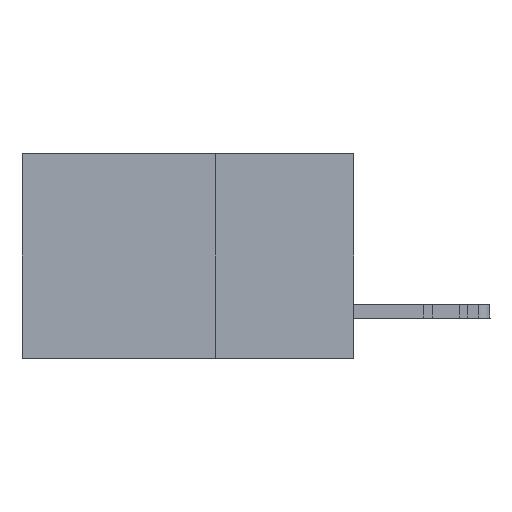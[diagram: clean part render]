
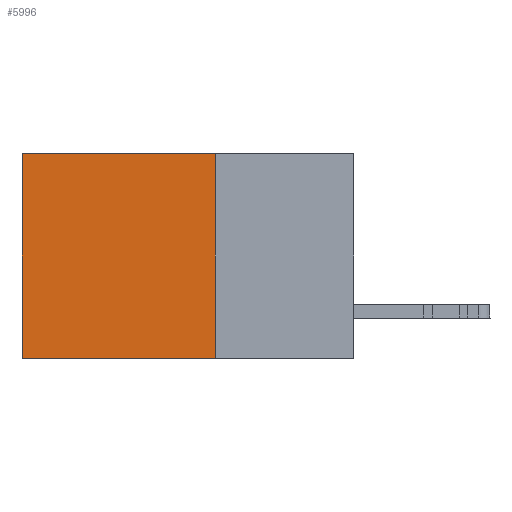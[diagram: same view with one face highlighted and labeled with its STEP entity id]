
A CAD part, left-side view. The second image highlights one B-rep face of the part: STEP entity #5996.
In plain terms, the highlighted planar face has unit normal (-1, 0, 0).
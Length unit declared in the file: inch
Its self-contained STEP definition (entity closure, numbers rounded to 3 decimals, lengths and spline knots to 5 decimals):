
#2182 = CARTESIAN_POINT ( 'NONE',  ( 0.2875, 0.25, -0.37 ) ) ;
#2769 = ORIENTED_EDGE ( 'NONE', *, *, #18118, .T. ) ;
#3696 = DIRECTION ( 'NONE',  ( 0., 0., -1. ) ) ;
#4790 = CARTESIAN_POINT ( 'NONE',  ( 0.2875, 0.25, 0. ) ) ;
#5996 = ADVANCED_FACE ( 'NONE', ( #18856 ), #25806, .F. ) ;
#6722 = CARTESIAN_POINT ( 'NONE',  ( 0.2875, 0.25, -0.37 ) ) ;
#7724 = DIRECTION ( 'NONE',  ( 0., 0., -1. ) ) ;
#10434 = CARTESIAN_POINT ( 'NONE',  ( 0.2875, 0.6, 0. ) ) ;
#10966 = VERTEX_POINT ( 'NONE', #10434 ) ;
#14449 = DIRECTION ( 'NONE',  ( 1., 0., 0. ) ) ;
#16374 = ORIENTED_EDGE ( 'NONE', *, *, #29642, .F. ) ;
#16858 = LINE ( 'NONE', #6722, #21499 ) ;
#17360 = ORIENTED_EDGE ( 'NONE', *, *, #20491, .F. ) ;
#18118 = EDGE_CURVE ( 'NONE', #10966, #45954, #29703, .T. ) ;
#18443 = CARTESIAN_POINT ( 'NONE',  ( 0.2875, 0.25, 0. ) ) ;
#18856 = FACE_OUTER_BOUND ( 'NONE', #36095, .T. ) ;
#20147 = CARTESIAN_POINT ( 'NONE',  ( 0.2875, 0.6, 0. ) ) ;
#20491 = EDGE_CURVE ( 'NONE', #46075, #43685, #34114, .T. ) ;
#21499 = VECTOR ( 'NONE', #36011, 39.37008 ) ;
#23917 = VECTOR ( 'NONE', #38473, 39.37008 ) ;
#24671 = CARTESIAN_POINT ( 'NONE',  ( 0.2875, 0.25, 0. ) ) ;
#25806 = PLANE ( 'NONE',  #40801 ) ;
#27270 = CARTESIAN_POINT ( 'NONE',  ( 0.2875, 0.6, -0.37 ) ) ;
#29283 = EDGE_CURVE ( 'NONE', #46075, #10966, #33214, .T. ) ;
#29642 = EDGE_CURVE ( 'NONE', #43685, #45954, #16858, .T. ) ;
#29703 = LINE ( 'NONE', #20147, #41432 ) ;
#31388 = DIRECTION ( 'NONE',  ( 0., 0., -1. ) ) ;
#33030 = ORIENTED_EDGE ( 'NONE', *, *, #29283, .T. ) ;
#33214 = LINE ( 'NONE', #4790, #23917 ) ;
#34114 = LINE ( 'NONE', #18443, #38155 ) ;
#36011 = DIRECTION ( 'NONE',  ( 0., 1., 0. ) ) ;
#36095 = EDGE_LOOP ( 'NONE', ( #2769, #16374, #17360, #33030 ) ) ;
#38155 = VECTOR ( 'NONE', #7724, 39.37008 ) ;
#38473 = DIRECTION ( 'NONE',  ( 0., 1., 0. ) ) ;
#40801 = AXIS2_PLACEMENT_3D ( 'NONE', #44550, #14449, #3696 ) ;
#41432 = VECTOR ( 'NONE', #31388, 39.37008 ) ;
#43685 = VERTEX_POINT ( 'NONE', #2182 ) ;
#44550 = CARTESIAN_POINT ( 'NONE',  ( 0.2875, 0.25, 0. ) ) ;
#45954 = VERTEX_POINT ( 'NONE', #27270 ) ;
#46075 = VERTEX_POINT ( 'NONE', #24671 ) ;
